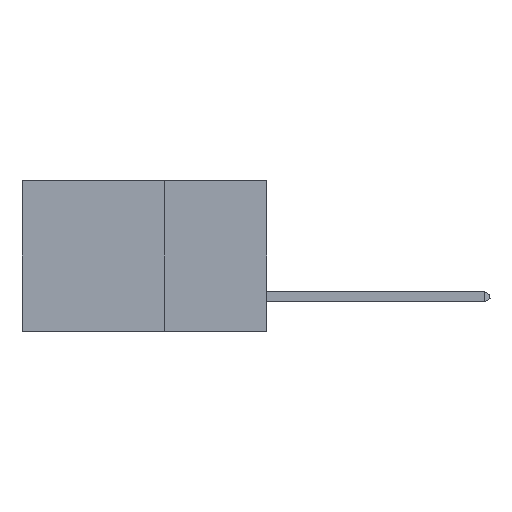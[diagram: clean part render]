
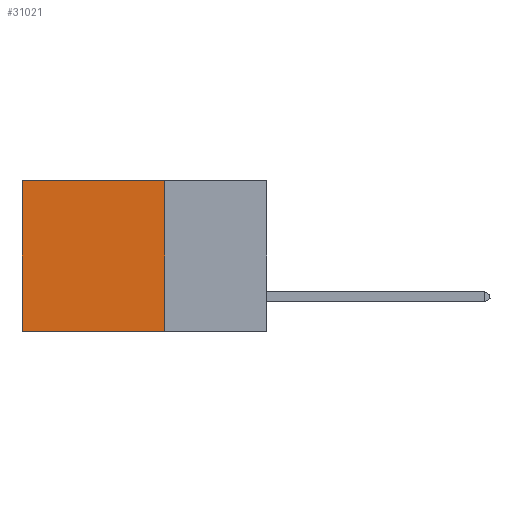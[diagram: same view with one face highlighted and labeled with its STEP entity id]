
A CAD part, left-side view. The second image highlights one B-rep face of the part: STEP entity #31021.
In plain terms, the highlighted planar face has unit normal (-1, 0, 0).
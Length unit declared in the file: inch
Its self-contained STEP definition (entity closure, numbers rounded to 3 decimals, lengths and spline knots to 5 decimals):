
#421 = VERTEX_POINT ( 'NONE', #13381 ) ;
#500 = CARTESIAN_POINT ( 'NONE',  ( 0.2875, 0.6, 0. ) ) ;
#504 = DIRECTION ( 'NONE',  ( 0., 0., -1. ) ) ;
#1127 = LINE ( 'NONE', #28988, #21948 ) ;
#1159 = AXIS2_PLACEMENT_3D ( 'NONE', #31737, #31602, #504 ) ;
#1708 = ORIENTED_EDGE ( 'NONE', *, *, #7453, .F. ) ;
#3843 = DIRECTION ( 'NONE',  ( 0., 1., 0. ) ) ;
#3956 = CARTESIAN_POINT ( 'NONE',  ( 0.2875, 0.25, -0.37 ) ) ;
#5024 = VECTOR ( 'NONE', #36070, 39.37008 ) ;
#6399 = CARTESIAN_POINT ( 'NONE',  ( 0.2875, 0.25, 0. ) ) ;
#7453 = EDGE_CURVE ( 'NONE', #421, #16580, #17913, .T. ) ;
#8801 = CARTESIAN_POINT ( 'NONE',  ( 0.2875, 0.25, 0. ) ) ;
#9764 = CARTESIAN_POINT ( 'NONE',  ( 0.2875, 0.6, -0.37 ) ) ;
#10427 = VECTOR ( 'NONE', #3843, 39.37008 ) ;
#13381 = CARTESIAN_POINT ( 'NONE',  ( 0.2875, 0.25, -0.37 ) ) ;
#15220 = DIRECTION ( 'NONE',  ( 0., 0., -1. ) ) ;
#16580 = VERTEX_POINT ( 'NONE', #9764 ) ;
#17337 = ORIENTED_EDGE ( 'NONE', *, *, #31575, .T. ) ;
#17913 = LINE ( 'NONE', #3956, #10427 ) ;
#19386 = FACE_OUTER_BOUND ( 'NONE', #34849, .T. ) ;
#19618 = ORIENTED_EDGE ( 'NONE', *, *, #29352, .F. ) ;
#20163 = PLANE ( 'NONE',  #1159 ) ;
#20729 = VERTEX_POINT ( 'NONE', #8801 ) ;
#21948 = VECTOR ( 'NONE', #15220, 39.37008 ) ;
#23055 = LINE ( 'NONE', #6399, #5024 ) ;
#25820 = ORIENTED_EDGE ( 'NONE', *, *, #26520, .T. ) ;
#26313 = DIRECTION ( 'NONE',  ( 0., 0., -1. ) ) ;
#26520 = EDGE_CURVE ( 'NONE', #20729, #26571, #23055, .T. ) ;
#26571 = VERTEX_POINT ( 'NONE', #500 ) ;
#27859 = VECTOR ( 'NONE', #26313, 39.37008 ) ;
#28774 = CARTESIAN_POINT ( 'NONE',  ( 0.2875, 0.25, 0. ) ) ;
#28988 = CARTESIAN_POINT ( 'NONE',  ( 0.2875, 0.6, 0. ) ) ;
#29352 = EDGE_CURVE ( 'NONE', #20729, #421, #29592, .T. ) ;
#29592 = LINE ( 'NONE', #28774, #27859 ) ;
#31021 = ADVANCED_FACE ( 'NONE', ( #19386 ), #20163, .F. ) ;
#31575 = EDGE_CURVE ( 'NONE', #26571, #16580, #1127, .T. ) ;
#31602 = DIRECTION ( 'NONE',  ( 1., 0., 0. ) ) ;
#31737 = CARTESIAN_POINT ( 'NONE',  ( 0.2875, 0.25, 0. ) ) ;
#34849 = EDGE_LOOP ( 'NONE', ( #17337, #1708, #19618, #25820 ) ) ;
#36070 = DIRECTION ( 'NONE',  ( 0., 1., 0. ) ) ;
